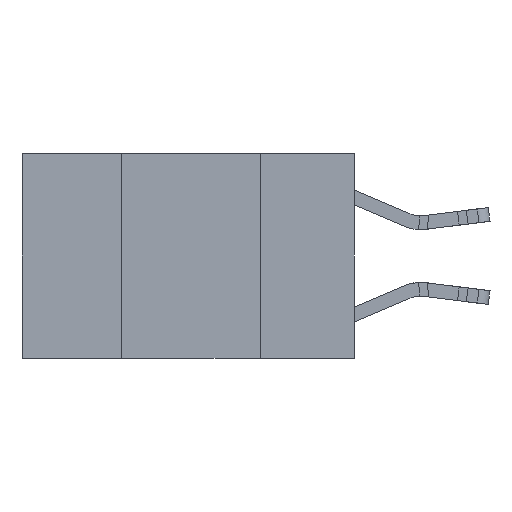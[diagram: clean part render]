
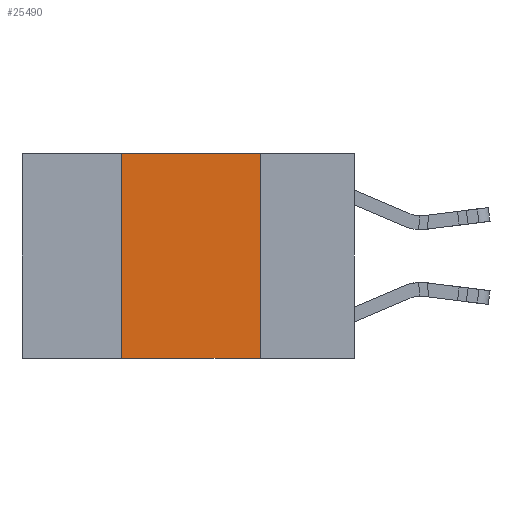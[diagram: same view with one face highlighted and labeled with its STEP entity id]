
A CAD part, left-side view. The second image highlights one B-rep face of the part: STEP entity #25490.
In plain terms, the highlighted planar face has unit normal (-1, 0, 0).
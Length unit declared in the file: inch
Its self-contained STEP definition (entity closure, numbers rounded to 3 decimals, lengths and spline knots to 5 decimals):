
#1290 = EDGE_LOOP ( 'NONE', ( #9360, #9414, #8998, #5105 ) ) ;
#1335 = AXIS2_PLACEMENT_3D ( 'NONE', #2546, #24347, #21356 ) ;
#2546 = CARTESIAN_POINT ( 'NONE',  ( 0., 0.6, 0. ) ) ;
#2684 = LINE ( 'NONE', #26260, #23209 ) ;
#5105 = ORIENTED_EDGE ( 'NONE', *, *, #6384, .T. ) ;
#6384 = EDGE_CURVE ( 'NONE', #19792, #10185, #20038, .T. ) ;
#7463 = DIRECTION ( 'NONE',  ( 0., -1., 0. ) ) ;
#8260 = CARTESIAN_POINT ( 'NONE',  ( 0., 0.42, 0. ) ) ;
#8324 = DIRECTION ( 'NONE',  ( 0., -1., 0. ) ) ;
#8445 = LINE ( 'NONE', #17854, #19883 ) ;
#8998 = ORIENTED_EDGE ( 'NONE', *, *, #17247, .F. ) ;
#9360 = ORIENTED_EDGE ( 'NONE', *, *, #20165, .F. ) ;
#9414 = ORIENTED_EDGE ( 'NONE', *, *, #15392, .F. ) ;
#9482 = FACE_OUTER_BOUND ( 'NONE', #1290, .T. ) ;
#9647 = VERTEX_POINT ( 'NONE', #8260 ) ;
#10185 = VERTEX_POINT ( 'NONE', #25022 ) ;
#12546 = LINE ( 'NONE', #26727, #25753 ) ;
#15392 = EDGE_CURVE ( 'NONE', #9647, #19534, #2684, .T. ) ;
#17247 = EDGE_CURVE ( 'NONE', #19792, #9647, #12546, .T. ) ;
#17490 = DIRECTION ( 'NONE',  ( 0., 0., 1. ) ) ;
#17854 = CARTESIAN_POINT ( 'NONE',  ( 0., 0.17, 0. ) ) ;
#18637 = CARTESIAN_POINT ( 'NONE',  ( 0., 0.42, -0.37 ) ) ;
#19534 = VERTEX_POINT ( 'NONE', #23914 ) ;
#19792 = VERTEX_POINT ( 'NONE', #18637 ) ;
#19883 = VECTOR ( 'NONE', #27231, 39.37008 ) ;
#20038 = LINE ( 'NONE', #29401, #28467 ) ;
#20165 = EDGE_CURVE ( 'NONE', #19534, #10185, #8445, .T. ) ;
#21046 = PLANE ( 'NONE',  #1335 ) ;
#21356 = DIRECTION ( 'NONE',  ( 0., 0., -1. ) ) ;
#23209 = VECTOR ( 'NONE', #7463, 39.37008 ) ;
#23914 = CARTESIAN_POINT ( 'NONE',  ( 0., 0.17, 0. ) ) ;
#24347 = DIRECTION ( 'NONE',  ( 1., 0., 0. ) ) ;
#25022 = CARTESIAN_POINT ( 'NONE',  ( 0., 0.17, -0.37 ) ) ;
#25490 = ADVANCED_FACE ( 'NONE', ( #9482 ), #21046, .F. ) ;
#25753 = VECTOR ( 'NONE', #17490, 39.37008 ) ;
#26260 = CARTESIAN_POINT ( 'NONE',  ( 0., 0.6, 0. ) ) ;
#26727 = CARTESIAN_POINT ( 'NONE',  ( 0., 0.42, 0. ) ) ;
#27231 = DIRECTION ( 'NONE',  ( 0., 0., -1. ) ) ;
#28467 = VECTOR ( 'NONE', #8324, 39.37008 ) ;
#29401 = CARTESIAN_POINT ( 'NONE',  ( 0., 0.6, -0.37 ) ) ;
